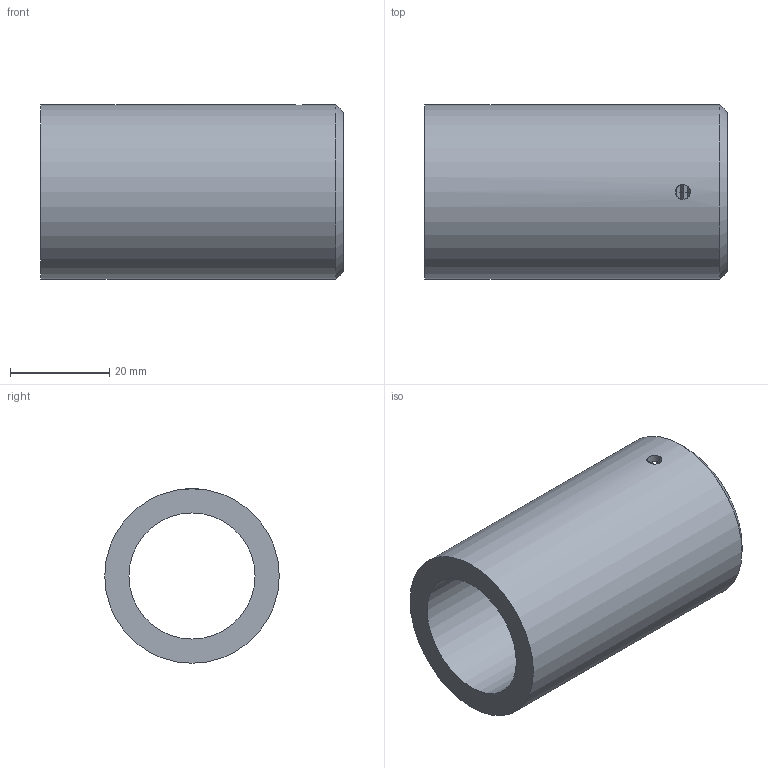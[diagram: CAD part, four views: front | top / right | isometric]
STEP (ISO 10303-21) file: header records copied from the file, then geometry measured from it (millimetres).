
FILE_DESCRIPTION(/* description */ (''),/* implementation_level */ '2;1');
FILE_NAME(/* name */ 'Barrel Nut Sleeve.step',/* time_stamp */ '2020-11-25T01:29:02-05:00',/* author */ (''),/* organization */ (''),/* preprocessor_version */ 'ST-DEVELOPER v18.1',/* originating_system */ 'Autodesk Translation Framework v9.3.0.1241',/* authorisation */ '');
FILE_SCHEMA (('AUTOMOTIVE_DESIGN { 1 0 10303 214 3 1 1 }'));
Length unit declared in the file: millimetre
Products named in the file (1): Barrel Nut Sleeve
Bounding box: 60.9 x 35.14 x 35.14 mm (x, y, z)
Volume: 24524.4 mm3; surface area: 13723.8 mm2
Topology: 1 solids, 1 shells, 85 faces, 220 edges, 137 vertices
Faces by surface type: cone 49, plane 19, cylinder 17
Full cylindrical faces by diameter (mm): 3 x1, 25.391 x1, 30.118 x1, 30.526 x1, 32.493 x4, 35.142 x1
Entity records: 3749 total; most frequent: CARTESIAN_POINT 1831, ORIENTED_EDGE 440, DIRECTION 323, EDGE_CURVE 220, VERTEX_POINT 137, AXIS2_PLACEMENT_3D 124, B_SPLINE_CURVE_WITH_KNOTS 94, EDGE_LOOP 89
